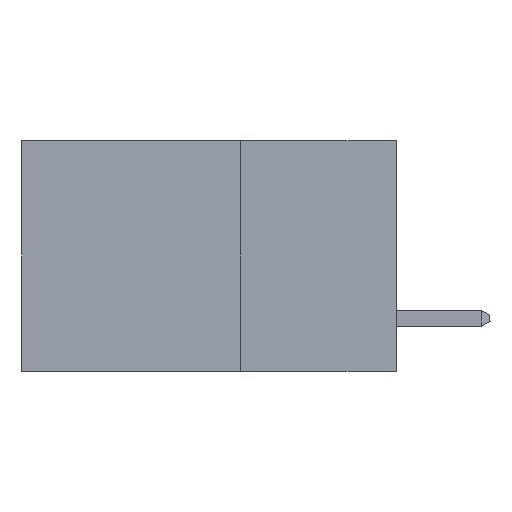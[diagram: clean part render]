
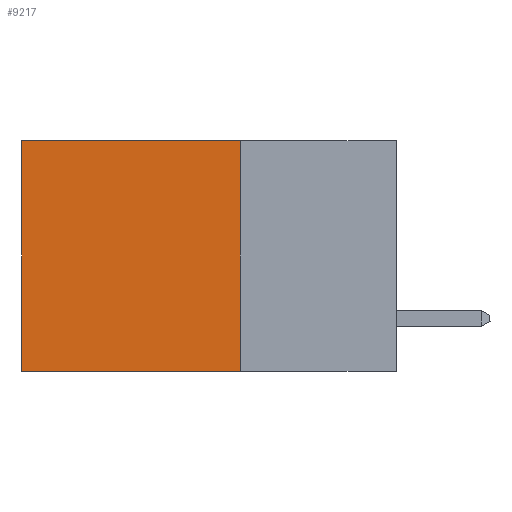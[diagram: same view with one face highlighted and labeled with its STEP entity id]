
A CAD part, left-side view. The second image highlights one B-rep face of the part: STEP entity #9217.
In plain terms, the highlighted planar face has unit normal (-1, 0, 0).
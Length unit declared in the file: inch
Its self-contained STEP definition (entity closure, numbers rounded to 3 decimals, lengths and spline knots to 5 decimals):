
#410 = ORIENTED_EDGE ( 'NONE', *, *, #2367, .T. ) ;
#423 = LINE ( 'NONE', #11772, #5835 ) ;
#1285 = CARTESIAN_POINT ( 'NONE',  ( 0.298, 0.25, 0. ) ) ;
#1287 = ORIENTED_EDGE ( 'NONE', *, *, #7619, .T. ) ;
#1406 = DIRECTION ( 'NONE',  ( 1., 0., 0. ) ) ;
#1608 = ORIENTED_EDGE ( 'NONE', *, *, #10919, .F. ) ;
#2033 = VECTOR ( 'NONE', #2206, 39.37008 ) ;
#2085 = VECTOR ( 'NONE', #11940, 39.37008 ) ;
#2206 = DIRECTION ( 'NONE',  ( 0., 0., -1. ) ) ;
#2367 = EDGE_CURVE ( 'NONE', #6762, #9423, #423, .T. ) ;
#2490 = VECTOR ( 'NONE', #5952, 39.37008 ) ;
#2494 = CARTESIAN_POINT ( 'NONE',  ( 0.298, 0.25, 0. ) ) ;
#4984 = LINE ( 'NONE', #2494, #2085 ) ;
#5407 = LINE ( 'NONE', #7889, #2490 ) ;
#5771 = DIRECTION ( 'NONE',  ( 0., 0., -1. ) ) ;
#5835 = VECTOR ( 'NONE', #5771, 39.37008 ) ;
#5952 = DIRECTION ( 'NONE',  ( 0., 1., 0. ) ) ;
#6207 = PLANE ( 'NONE',  #10809 ) ;
#6565 = VERTEX_POINT ( 'NONE', #7716 ) ;
#6714 = CARTESIAN_POINT ( 'NONE',  ( 0.298, 0.25, -0.37 ) ) ;
#6762 = VERTEX_POINT ( 'NONE', #11832 ) ;
#7200 = CARTESIAN_POINT ( 'NONE',  ( 0.298, 0.25, 0. ) ) ;
#7619 = EDGE_CURVE ( 'NONE', #6565, #6762, #4984, .T. ) ;
#7716 = CARTESIAN_POINT ( 'NONE',  ( 0.298, 0.25, 0. ) ) ;
#7889 = CARTESIAN_POINT ( 'NONE',  ( 0.298, 0.25, -0.37 ) ) ;
#8168 = DIRECTION ( 'NONE',  ( 0., 0., -1. ) ) ;
#9217 = ADVANCED_FACE ( 'NONE', ( #11945 ), #6207, .F. ) ;
#9423 = VERTEX_POINT ( 'NONE', #12049 ) ;
#9953 = VERTEX_POINT ( 'NONE', #6714 ) ;
#10098 = EDGE_LOOP ( 'NONE', ( #410, #10578, #1608, #1287 ) ) ;
#10167 = EDGE_CURVE ( 'NONE', #9953, #9423, #5407, .T. ) ;
#10578 = ORIENTED_EDGE ( 'NONE', *, *, #10167, .F. ) ;
#10809 = AXIS2_PLACEMENT_3D ( 'NONE', #7200, #1406, #8168 ) ;
#10919 = EDGE_CURVE ( 'NONE', #6565, #9953, #12054, .T. ) ;
#11772 = CARTESIAN_POINT ( 'NONE',  ( 0.298, 0.6, 0. ) ) ;
#11832 = CARTESIAN_POINT ( 'NONE',  ( 0.298, 0.6, 0. ) ) ;
#11940 = DIRECTION ( 'NONE',  ( 0., 1., 0. ) ) ;
#11945 = FACE_OUTER_BOUND ( 'NONE', #10098, .T. ) ;
#12049 = CARTESIAN_POINT ( 'NONE',  ( 0.298, 0.6, -0.37 ) ) ;
#12054 = LINE ( 'NONE', #1285, #2033 ) ;
